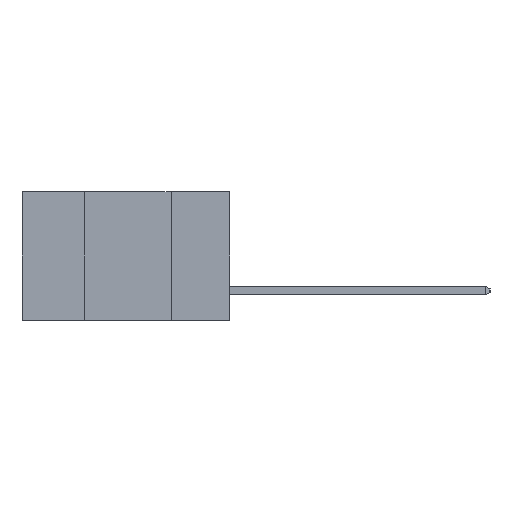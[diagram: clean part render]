
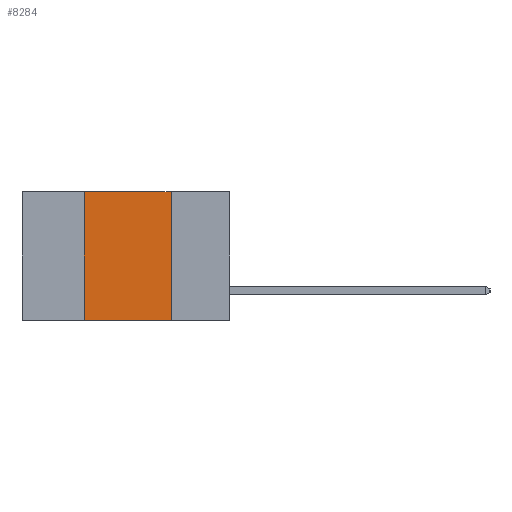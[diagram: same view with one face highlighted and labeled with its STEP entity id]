
A CAD part, left-side view. The second image highlights one B-rep face of the part: STEP entity #8284.
In plain terms, the highlighted planar face has unit normal (-1, 0, 0).
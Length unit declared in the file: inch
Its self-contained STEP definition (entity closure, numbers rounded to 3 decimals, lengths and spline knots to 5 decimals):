
#220 = LINE ( 'NONE', #2338, #6825 ) ;
#370 = EDGE_CURVE ( 'NONE', #2705, #5594, #5261, .T. ) ;
#2049 = DIRECTION ( 'NONE',  ( 0., -1., 0. ) ) ;
#2338 = CARTESIAN_POINT ( 'NONE',  ( 0., 0.6, 0. ) ) ;
#2376 = VECTOR ( 'NONE', #3961, 39.37008 ) ;
#2476 = ORIENTED_EDGE ( 'NONE', *, *, #370, .T. ) ;
#2705 = VERTEX_POINT ( 'NONE', #5379 ) ;
#3015 = DIRECTION ( 'NONE',  ( 0., 0., -1. ) ) ;
#3776 = EDGE_LOOP ( 'NONE', ( #7304, #7037, #4819, #2476 ) ) ;
#3961 = DIRECTION ( 'NONE',  ( 0., 0., 1. ) ) ;
#4819 = ORIENTED_EDGE ( 'NONE', *, *, #10166, .F. ) ;
#4945 = VERTEX_POINT ( 'NONE', #5537 ) ;
#5215 = CARTESIAN_POINT ( 'NONE',  ( 0., 0.42, 0. ) ) ;
#5261 = LINE ( 'NONE', #7424, #9088 ) ;
#5379 = CARTESIAN_POINT ( 'NONE',  ( 0., 0.42, -0.37 ) ) ;
#5537 = CARTESIAN_POINT ( 'NONE',  ( 0., 0.17, 0. ) ) ;
#5594 = VERTEX_POINT ( 'NONE', #6473 ) ;
#6381 = EDGE_CURVE ( 'NONE', #4945, #5594, #6630, .T. ) ;
#6414 = VERTEX_POINT ( 'NONE', #5215 ) ;
#6473 = CARTESIAN_POINT ( 'NONE',  ( 0., 0.17, -0.37 ) ) ;
#6630 = LINE ( 'NONE', #6695, #7126 ) ;
#6683 = LINE ( 'NONE', #9748, #2376 ) ;
#6695 = CARTESIAN_POINT ( 'NONE',  ( 0., 0.17, -0.37 ) ) ;
#6825 = VECTOR ( 'NONE', #2049, 39.37008 ) ;
#7037 = ORIENTED_EDGE ( 'NONE', *, *, #9078, .F. ) ;
#7126 = VECTOR ( 'NONE', #3015, 39.37008 ) ;
#7304 = ORIENTED_EDGE ( 'NONE', *, *, #6381, .F. ) ;
#7424 = CARTESIAN_POINT ( 'NONE',  ( 0., 0.6, -0.37 ) ) ;
#7624 = AXIS2_PLACEMENT_3D ( 'NONE', #7902, #8960, #8544 ) ;
#7902 = CARTESIAN_POINT ( 'NONE',  ( 0., 0.6, 0. ) ) ;
#8284 = ADVANCED_FACE ( 'NONE', ( #9506 ), #9320, .F. ) ;
#8544 = DIRECTION ( 'NONE',  ( 0., 0., -1. ) ) ;
#8960 = DIRECTION ( 'NONE',  ( 1., 0., 0. ) ) ;
#9078 = EDGE_CURVE ( 'NONE', #6414, #4945, #220, .T. ) ;
#9088 = VECTOR ( 'NONE', #9346, 39.37008 ) ;
#9320 = PLANE ( 'NONE',  #7624 ) ;
#9346 = DIRECTION ( 'NONE',  ( 0., -1., 0. ) ) ;
#9506 = FACE_OUTER_BOUND ( 'NONE', #3776, .T. ) ;
#9748 = CARTESIAN_POINT ( 'NONE',  ( 0., 0.42, -0.37 ) ) ;
#10166 = EDGE_CURVE ( 'NONE', #2705, #6414, #6683, .T. ) ;
